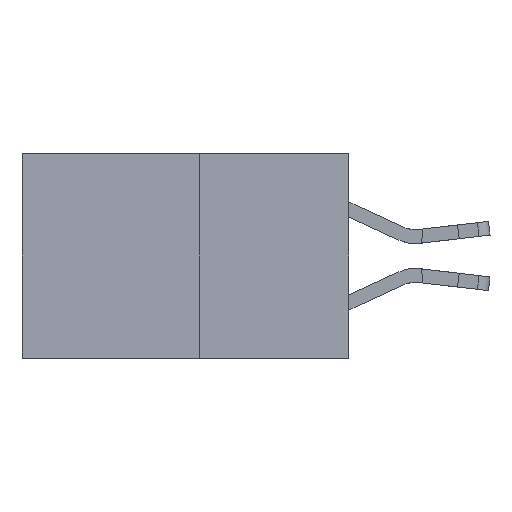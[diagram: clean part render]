
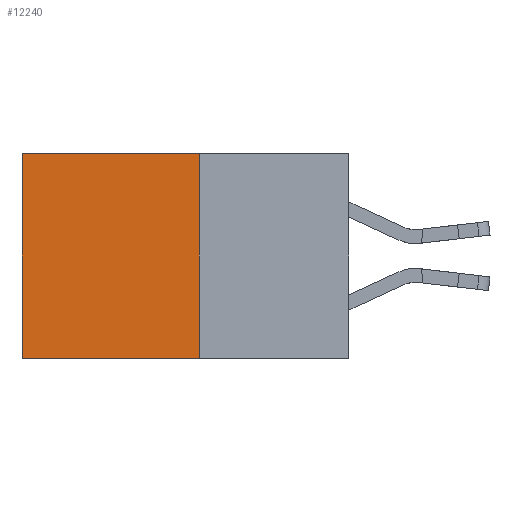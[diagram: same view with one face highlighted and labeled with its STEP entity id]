
A CAD part, left-side view. The second image highlights one B-rep face of the part: STEP entity #12240.
In plain terms, the highlighted planar face has unit normal (-1, 0, 0).
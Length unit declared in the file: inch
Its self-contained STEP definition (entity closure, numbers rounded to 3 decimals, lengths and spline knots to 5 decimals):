
#3 = DIRECTION ( 'NONE',  ( 0., 0., -1. ) ) ;
#354 = CARTESIAN_POINT ( 'NONE',  ( 0.277, 0.27, -0.37 ) ) ;
#1371 = DIRECTION ( 'NONE',  ( 0., 0., -1. ) ) ;
#1375 = ORIENTED_EDGE ( 'NONE', *, *, #16957, .F. ) ;
#1430 = CARTESIAN_POINT ( 'NONE',  ( 0.277, 0.27, -0.37 ) ) ;
#1536 = VECTOR ( 'NONE', #15119, 39.37008 ) ;
#2468 = VECTOR ( 'NONE', #7045, 39.37008 ) ;
#2620 = EDGE_CURVE ( 'NONE', #8629, #18106, #8909, .T. ) ;
#2873 = CARTESIAN_POINT ( 'NONE',  ( 0.277, 0.27, 0. ) ) ;
#2942 = FACE_OUTER_BOUND ( 'NONE', #10049, .T. ) ;
#3355 = DIRECTION ( 'NONE',  ( 0., 1., 0. ) ) ;
#3564 = CARTESIAN_POINT ( 'NONE',  ( 0.277, 0.27, 0. ) ) ;
#4198 = ORIENTED_EDGE ( 'NONE', *, *, #17261, .F. ) ;
#4554 = VERTEX_POINT ( 'NONE', #17793 ) ;
#5536 = CARTESIAN_POINT ( 'NONE',  ( 0.277, 0.27, -0.37 ) ) ;
#6610 = CARTESIAN_POINT ( 'NONE',  ( 0.277, 0.59, 0. ) ) ;
#7045 = DIRECTION ( 'NONE',  ( 0., 0., -1. ) ) ;
#7458 = PLANE ( 'NONE',  #13677 ) ;
#7574 = VERTEX_POINT ( 'NONE', #354 ) ;
#8310 = LINE ( 'NONE', #17673, #15787 ) ;
#8629 = VERTEX_POINT ( 'NONE', #2873 ) ;
#8908 = DIRECTION ( 'NONE',  ( 1., 0., 0. ) ) ;
#8909 = LINE ( 'NONE', #3564, #16398 ) ;
#10049 = EDGE_LOOP ( 'NONE', ( #13155, #4198, #1375, #16880 ) ) ;
#10352 = LINE ( 'NONE', #5536, #2468 ) ;
#12240 = ADVANCED_FACE ( 'NONE', ( #2942 ), #7458, .F. ) ;
#13155 = ORIENTED_EDGE ( 'NONE', *, *, #16426, .T. ) ;
#13430 = LINE ( 'NONE', #16532, #1536 ) ;
#13677 = AXIS2_PLACEMENT_3D ( 'NONE', #1430, #8908, #3 ) ;
#15119 = DIRECTION ( 'NONE',  ( 0., 1., 0. ) ) ;
#15787 = VECTOR ( 'NONE', #1371, 39.37008 ) ;
#16398 = VECTOR ( 'NONE', #3355, 39.37008 ) ;
#16426 = EDGE_CURVE ( 'NONE', #18106, #4554, #8310, .T. ) ;
#16532 = CARTESIAN_POINT ( 'NONE',  ( 0.277, 0.27, -0.37 ) ) ;
#16880 = ORIENTED_EDGE ( 'NONE', *, *, #2620, .T. ) ;
#16957 = EDGE_CURVE ( 'NONE', #8629, #7574, #10352, .T. ) ;
#17261 = EDGE_CURVE ( 'NONE', #7574, #4554, #13430, .T. ) ;
#17673 = CARTESIAN_POINT ( 'NONE',  ( 0.277, 0.59, -0.37 ) ) ;
#17793 = CARTESIAN_POINT ( 'NONE',  ( 0.277, 0.59, -0.37 ) ) ;
#18106 = VERTEX_POINT ( 'NONE', #6610 ) ;
